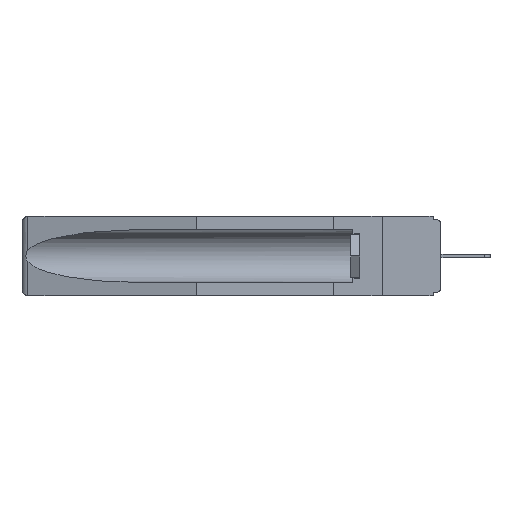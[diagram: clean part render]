
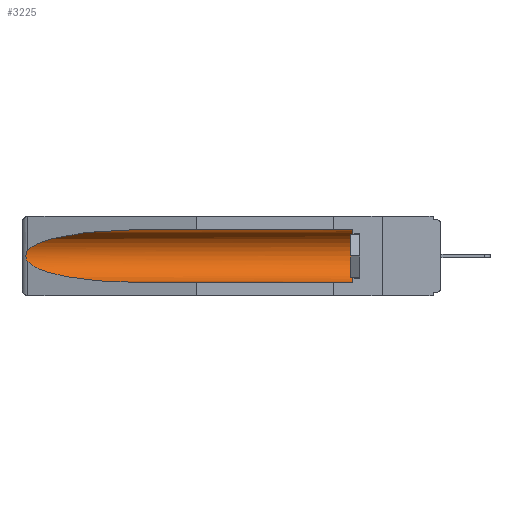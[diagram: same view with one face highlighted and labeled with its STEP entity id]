
A CAD part, left-side view. The second image highlights one B-rep face of the part: STEP entity #3225.
In plain terms, the highlighted cylindrical face has radius 2.857 mm (diameter 5.715 mm), a partial arc.
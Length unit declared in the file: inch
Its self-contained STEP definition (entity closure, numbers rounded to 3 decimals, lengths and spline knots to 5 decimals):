
#550 = LINE ( 'NONE', #4703, #4394 ) ;
#626 = CARTESIAN_POINT ( 'NONE',  ( 0.25451, 1.48313, -0.09465 ) ) ;
#810 = CARTESIAN_POINT ( 'NONE',  ( 0.26537, 1.52718, -0.14972 ) ) ;
#951 = CARTESIAN_POINT ( 'NONE',  ( 0.26537, 1.52718, -0.14972 ) ) ;
#1158 = CYLINDRICAL_SURFACE ( 'NONE', #1257, 0.1125 ) ;
#1257 = AXIS2_PLACEMENT_3D ( 'NONE', #15035, #3756, #9308 ) ;
#1353 = DIRECTION ( 'NONE',  ( 0., -1., 0. ) ) ;
#1585 = VERTEX_POINT ( 'NONE', #8113 ) ;
#2702 = CARTESIAN_POINT ( 'NONE',  ( 0.2673, 1.53269, -0.17917 ) ) ;
#2782 = EDGE_CURVE ( 'NONE', #11720, #13267, #7513, .T. ) ;
#3125 = EDGE_CURVE ( 'NONE', #1585, #13978, #5961, .T. ) ;
#3142 = DIRECTION ( 'NONE',  ( 0., 1., 0. ) ) ;
#3225 = ADVANCED_FACE ( 'NONE', ( #9110 ), #1158, .F. ) ;
#3239 = CARTESIAN_POINT ( 'NONE',  ( 0.26597, 1.5296, -0.19026 ) ) ;
#3756 = DIRECTION ( 'NONE',  ( 0., 1., 0. ) ) ;
#3965 = EDGE_CURVE ( 'NONE', #11939, #13978, #17105, .T. ) ;
#4006 = EDGE_CURVE ( 'NONE', #7122, #11720, #550, .T. ) ;
#4262 = CARTESIAN_POINT ( 'NONE',  ( 0.26537, 1.52718, -0.19328 ) ) ;
#4394 = VECTOR ( 'NONE', #3142, 39.37008 ) ;
#4703 = CARTESIAN_POINT ( 'NONE',  ( 0.155, -0.30754, -0.059 ) ) ;
#5433 = CARTESIAN_POINT ( 'NONE',  ( 0.26537, 1.52718, -0.14972 ) ) ;
#5685 = DIRECTION ( 'NONE',  ( 0., 0., 1. ) ) ;
#5961 = LINE ( 'NONE', #6338, #13665 ) ;
#6093 = CARTESIAN_POINT ( 'NONE',  ( 0.25451, 1.48313, -0.24835 ) ) ;
#6180 = CARTESIAN_POINT ( 'NONE',  ( 0.21114, 1.30732, -0.284 ) ) ;
#6338 = CARTESIAN_POINT ( 'NONE',  ( 0.155, -0.30754, -0.284 ) ) ;
#6429 = CARTESIAN_POINT ( 'NONE',  ( 0.26597, 1.52961, -0.15275 ) ) ;
#6973 = CARTESIAN_POINT ( 'NONE',  ( 0.155, 0.126, -0.1715 ) ) ;
#7122 = VERTEX_POINT ( 'NONE', #12582 ) ;
#7148 = ORIENTED_EDGE ( 'NONE', *, *, #9194, .T. ) ;
#7513 =( BOUNDED_CURVE ( )  B_SPLINE_CURVE ( 3, ( #9038, #14678, #626, #5433 ),
 .UNSPECIFIED., .F., .F. ) 
 B_SPLINE_CURVE_WITH_KNOTS ( ( 4, 4 ),
 ( 4.71239, 6.08839 ),
 .UNSPECIFIED. ) 
 CURVE ( )  GEOMETRIC_REPRESENTATION_ITEM ( )  RATIONAL_B_SPLINE_CURVE ( ( 1., 0.848, 0.848, 1. ) ) 
 REPRESENTATION_ITEM ( '' )  );
#8113 = CARTESIAN_POINT ( 'NONE',  ( 0.155, 0.126, -0.284 ) ) ;
#8344 = CARTESIAN_POINT ( 'NONE',  ( 0.26655, 1.53094, -0.18657 ) ) ;
#8739 = DIRECTION ( 'NONE',  ( 0., 1., 0. ) ) ;
#9038 = CARTESIAN_POINT ( 'NONE',  ( 0.155, 1.07973, -0.059 ) ) ;
#9110 = FACE_OUTER_BOUND ( 'NONE', #13866, .T. ) ;
#9194 = EDGE_CURVE ( 'NONE', #1585, #7122, #9256, .T. ) ;
#9256 = CIRCLE ( 'NONE', #15760, 0.1125 ) ;
#9308 = DIRECTION ( 'NONE',  ( 0., 0., 1. ) ) ;
#10025 = CARTESIAN_POINT ( 'NONE',  ( 0.155, 1.07973, -0.284 ) ) ;
#10577 = ORIENTED_EDGE ( 'NONE', *, *, #3965, .T. ) ;
#10698 = CARTESIAN_POINT ( 'NONE',  ( 0.2673, 1.5327, -0.16383 ) ) ;
#11720 = VERTEX_POINT ( 'NONE', #17241 ) ;
#11939 = VERTEX_POINT ( 'NONE', #15346 ) ;
#12010 = B_SPLINE_CURVE_WITH_KNOTS ( 'NONE', 3,
 ( #810, #6429, #17747, #10698, #12523, #15375, #2702, #8344, #3239, #12961 ),
 .UNSPECIFIED., .F., .F.,
 ( 4, 2, 2, 2, 4 ),
 ( 0., 0.00029, 0.00058, 0.00087, 0.00117 ),
 .UNSPECIFIED. ) ;
#12067 = ORIENTED_EDGE ( 'NONE', *, *, #3125, .F. ) ;
#12523 = CARTESIAN_POINT ( 'NONE',  ( 0.2675, 1.53308, -0.16763 ) ) ;
#12582 = CARTESIAN_POINT ( 'NONE',  ( 0.155, 0.126, -0.059 ) ) ;
#12914 = EDGE_CURVE ( 'NONE', #13267, #11939, #12010, .T. ) ;
#12961 = CARTESIAN_POINT ( 'NONE',  ( 0.26537, 1.52718, -0.19328 ) ) ;
#13267 = VERTEX_POINT ( 'NONE', #951 ) ;
#13665 = VECTOR ( 'NONE', #8739, 39.37008 ) ;
#13866 = EDGE_LOOP ( 'NONE', ( #14072, #15311, #10577, #12067, #7148, #16219 ) ) ;
#13978 = VERTEX_POINT ( 'NONE', #10025 ) ;
#14072 = ORIENTED_EDGE ( 'NONE', *, *, #2782, .T. ) ;
#14678 = CARTESIAN_POINT ( 'NONE',  ( 0.21114, 1.30732, -0.059 ) ) ;
#15035 = CARTESIAN_POINT ( 'NONE',  ( 0.155, -0.30754, -0.1715 ) ) ;
#15311 = ORIENTED_EDGE ( 'NONE', *, *, #12914, .T. ) ;
#15346 = CARTESIAN_POINT ( 'NONE',  ( 0.26537, 1.52718, -0.19328 ) ) ;
#15375 = CARTESIAN_POINT ( 'NONE',  ( 0.2675, 1.53308, -0.17534 ) ) ;
#15760 = AXIS2_PLACEMENT_3D ( 'NONE', #6973, #1353, #5685 ) ;
#16015 = CARTESIAN_POINT ( 'NONE',  ( 0.155, 1.07973, -0.284 ) ) ;
#16219 = ORIENTED_EDGE ( 'NONE', *, *, #4006, .T. ) ;
#17105 =( BOUNDED_CURVE ( )  B_SPLINE_CURVE ( 3, ( #4262, #6093, #6180, #16015 ),
 .UNSPECIFIED., .F., .F. ) 
 B_SPLINE_CURVE_WITH_KNOTS ( ( 4, 4 ),
 ( 0.1948, 1.5708 ),
 .UNSPECIFIED. ) 
 CURVE ( )  GEOMETRIC_REPRESENTATION_ITEM ( )  RATIONAL_B_SPLINE_CURVE ( ( 1., 0.848, 0.848, 1. ) ) 
 REPRESENTATION_ITEM ( '' )  );
#17241 = CARTESIAN_POINT ( 'NONE',  ( 0.155, 1.07973, -0.059 ) ) ;
#17747 = CARTESIAN_POINT ( 'NONE',  ( 0.26654, 1.53092, -0.15636 ) ) ;
